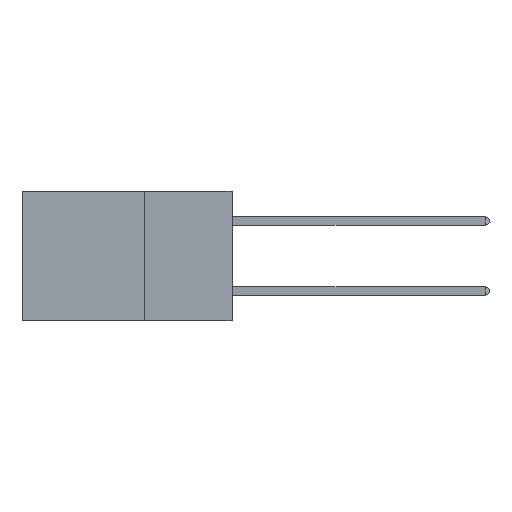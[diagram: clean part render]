
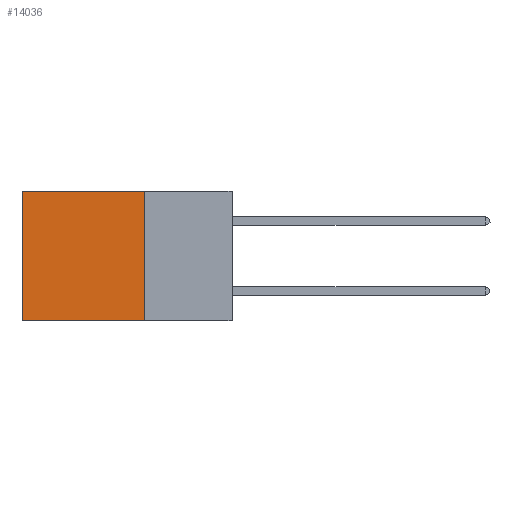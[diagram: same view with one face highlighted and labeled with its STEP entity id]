
A CAD part, left-side view. The second image highlights one B-rep face of the part: STEP entity #14036.
In plain terms, the highlighted planar face has unit normal (-1, 0, 0).
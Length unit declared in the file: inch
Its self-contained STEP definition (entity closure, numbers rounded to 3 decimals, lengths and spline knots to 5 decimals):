
#167 = ORIENTED_EDGE ( 'NONE', *, *, #11735, .T. ) ;
#673 = DIRECTION ( 'NONE',  ( 0., 1., 0. ) ) ;
#2269 = ORIENTED_EDGE ( 'NONE', *, *, #12693, .F. ) ;
#2529 = PLANE ( 'NONE',  #7757 ) ;
#2627 = VECTOR ( 'NONE', #15287, 39.37008 ) ;
#3642 = CARTESIAN_POINT ( 'NONE',  ( 0.2875, 0.25, -0.37 ) ) ;
#4091 = VERTEX_POINT ( 'NONE', #9851 ) ;
#4669 = CARTESIAN_POINT ( 'NONE',  ( 0.2875, 0.25, 0. ) ) ;
#4902 = VECTOR ( 'NONE', #673, 39.37008 ) ;
#5017 = EDGE_LOOP ( 'NONE', ( #167, #2269, #18558, #15233 ) ) ;
#5063 = VERTEX_POINT ( 'NONE', #4669 ) ;
#5501 = CARTESIAN_POINT ( 'NONE',  ( 0.2875, 0.6, 0. ) ) ;
#7145 = EDGE_CURVE ( 'NONE', #5063, #15158, #8563, .T. ) ;
#7337 = FACE_OUTER_BOUND ( 'NONE', #5017, .T. ) ;
#7532 = CARTESIAN_POINT ( 'NONE',  ( 0.2875, 0.25, 0. ) ) ;
#7757 = AXIS2_PLACEMENT_3D ( 'NONE', #18187, #8792, #12032 ) ;
#8563 = LINE ( 'NONE', #13799, #2627 ) ;
#8792 = DIRECTION ( 'NONE',  ( 1., 0., 0. ) ) ;
#9851 = CARTESIAN_POINT ( 'NONE',  ( 0.2875, 0.6, -0.37 ) ) ;
#11082 = DIRECTION ( 'NONE',  ( 0., 0., -1. ) ) ;
#11616 = CARTESIAN_POINT ( 'NONE',  ( 0.2875, 0.25, -0.37 ) ) ;
#11657 = EDGE_CURVE ( 'NONE', #5063, #18779, #18451, .T. ) ;
#11735 = EDGE_CURVE ( 'NONE', #18779, #4091, #18675, .T. ) ;
#12032 = DIRECTION ( 'NONE',  ( 0., 0., -1. ) ) ;
#12693 = EDGE_CURVE ( 'NONE', #15158, #4091, #20099, .T. ) ;
#13792 = DIRECTION ( 'NONE',  ( 0., 1., 0. ) ) ;
#13799 = CARTESIAN_POINT ( 'NONE',  ( 0.2875, 0.25, 0. ) ) ;
#14036 = ADVANCED_FACE ( 'NONE', ( #7337 ), #2529, .F. ) ;
#15158 = VERTEX_POINT ( 'NONE', #3642 ) ;
#15233 = ORIENTED_EDGE ( 'NONE', *, *, #11657, .T. ) ;
#15287 = DIRECTION ( 'NONE',  ( 0., 0., -1. ) ) ;
#16230 = VECTOR ( 'NONE', #13792, 39.37008 ) ;
#18187 = CARTESIAN_POINT ( 'NONE',  ( 0.2875, 0.25, 0. ) ) ;
#18451 = LINE ( 'NONE', #7532, #16230 ) ;
#18558 = ORIENTED_EDGE ( 'NONE', *, *, #7145, .F. ) ;
#18675 = LINE ( 'NONE', #18893, #19170 ) ;
#18779 = VERTEX_POINT ( 'NONE', #5501 ) ;
#18893 = CARTESIAN_POINT ( 'NONE',  ( 0.2875, 0.6, 0. ) ) ;
#19170 = VECTOR ( 'NONE', #11082, 39.37008 ) ;
#20099 = LINE ( 'NONE', #11616, #4902 ) ;
